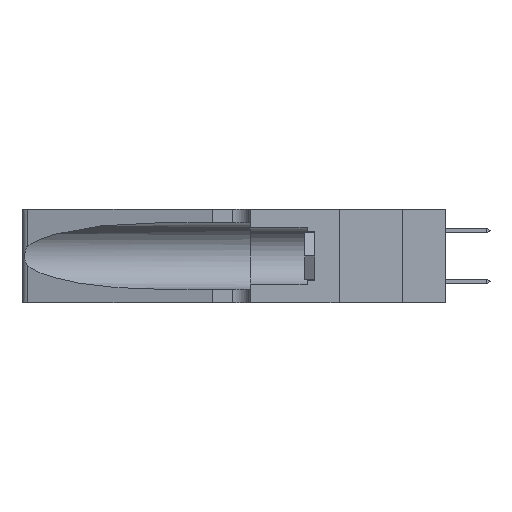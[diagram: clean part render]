
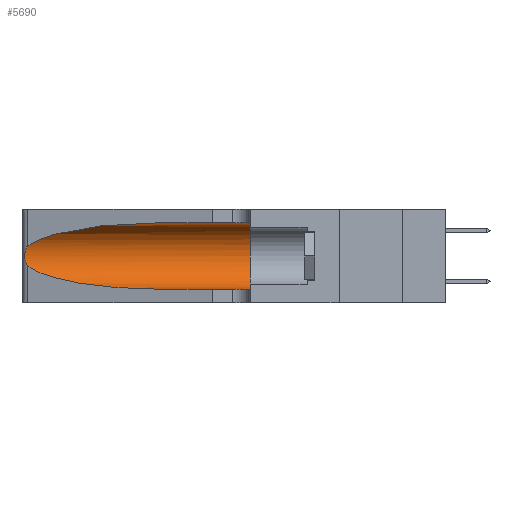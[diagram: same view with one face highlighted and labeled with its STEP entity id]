
A CAD part, left-side view. The second image highlights one B-rep face of the part: STEP entity #5690.
In plain terms, the highlighted cylindrical face has radius 3.308 mm (diameter 6.617 mm), a partial arc.
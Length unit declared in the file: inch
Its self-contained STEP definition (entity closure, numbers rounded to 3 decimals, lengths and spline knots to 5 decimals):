
#400 = VECTOR ( 'NONE', #7808, 39.37008 ) ;
#1198 = CARTESIAN_POINT ( 'NONE',  ( 0.1305, 0.72297, 0.31525 ) ) ;
#2010 = DIRECTION ( 'NONE',  ( 0., -1., 0. ) ) ;
#2629 = CYLINDRICAL_SURFACE ( 'NONE', #35287, 0.13025 ) ;
#2795 = CARTESIAN_POINT ( 'NONE',  ( 0.25555, 1.22994, 0.2215 ) ) ;
#2952 = CARTESIAN_POINT ( 'NONE',  ( 0.26017, 1.23833, 0.17102 ) ) ;
#3348 = ORIENTED_EDGE ( 'NONE', *, *, #23739, .T. ) ;
#4155 = CARTESIAN_POINT ( 'NONE',  ( 0.1305, 1.61858, 0.185 ) ) ;
#5389 = CARTESIAN_POINT ( 'NONE',  ( 0.18966, 0.96281, 0.05475 ) ) ;
#5690 = ADVANCED_FACE ( 'NONE', ( #29784 ), #2629, .F. ) ;
#6075 = DIRECTION ( 'NONE',  ( 0., 1., 0. ) ) ;
#6386 =( BOUNDED_CURVE ( )  B_SPLINE_CURVE ( 3, ( #1198, #14910, #35188, #15056 ),
 .UNSPECIFIED., .F., .T. ) 
 B_SPLINE_CURVE_WITH_KNOTS ( ( 4, 4 ),
 ( 1.5708, 2.84003 ),
 .UNSPECIFIED. ) 
 CURVE ( )  GEOMETRIC_REPRESENTATION_ITEM ( )  RATIONAL_B_SPLINE_CURVE ( ( 1., 0.87, 0.87, 1. ) ) 
 REPRESENTATION_ITEM ( '' )  );
#6492 = CARTESIAN_POINT ( 'NONE',  ( 0.25789, 1.23486, 0.15765 ) ) ;
#7808 = DIRECTION ( 'NONE',  ( 0., -1., 0. ) ) ;
#9900 = CARTESIAN_POINT ( 'NONE',  ( 0.25555, 1.22993, 0.14849 ) ) ;
#12673 = CARTESIAN_POINT ( 'NONE',  ( 0.1305, 0.35, 0.31525 ) ) ;
#12881 = VERTEX_POINT ( 'NONE', #30099 ) ;
#13112 = LINE ( 'NONE', #19233, #38848 ) ;
#14059 = ORIENTED_EDGE ( 'NONE', *, *, #23869, .T. ) ;
#14910 = CARTESIAN_POINT ( 'NONE',  ( 0.18966, 0.96281, 0.31525 ) ) ;
#15056 = CARTESIAN_POINT ( 'NONE',  ( 0.25487, 1.22718, 0.22369 ) ) ;
#16601 = CARTESIAN_POINT ( 'NONE',  ( 0.25787, 1.23484, 0.2124 ) ) ;
#16958 = AXIS2_PLACEMENT_3D ( 'NONE', #26392, #6075, #29749 ) ;
#17268 = ORIENTED_EDGE ( 'NONE', *, *, #38435, .T. ) ;
#17328 = VERTEX_POINT ( 'NONE', #18213 ) ;
#17730 = DIRECTION ( 'NONE',  ( 0., 0., -1. ) ) ;
#18213 = CARTESIAN_POINT ( 'NONE',  ( 0.25487, 1.22718, 0.14631 ) ) ;
#18695 = VERTEX_POINT ( 'NONE', #31154 ) ;
#18898 = CARTESIAN_POINT ( 'NONE',  ( 0.25487, 1.22718, 0.14631 ) ) ;
#19001 = CIRCLE ( 'NONE', #16958, 0.13025 ) ;
#19233 = CARTESIAN_POINT ( 'NONE',  ( 0.1305, 1.61858, 0.31525 ) ) ;
#19985 = CARTESIAN_POINT ( 'NONE',  ( 0.26018, 1.23835, 0.19895 ) ) ;
#20407 = VERTEX_POINT ( 'NONE', #39765 ) ;
#20425 = ORIENTED_EDGE ( 'NONE', *, *, #37039, .T. ) ;
#21340 = VERTEX_POINT ( 'NONE', #38724 ) ;
#21451 = EDGE_CURVE ( 'NONE', #12881, #41234, #13112, .T. ) ;
#23393 = CARTESIAN_POINT ( 'NONE',  ( 0.26075, 1.23896, 0.178 ) ) ;
#23739 = EDGE_CURVE ( 'NONE', #20407, #21340, #35453, .T. ) ;
#23869 = EDGE_CURVE ( 'NONE', #12881, #18695, #6386, .T. ) ;
#24214 = EDGE_LOOP ( 'NONE', ( #14059, #17268, #20425, #3348, #43461, #37735 ) ) ;
#24518 = DIRECTION ( 'NONE',  ( 0., -1., 0. ) ) ;
#26392 = CARTESIAN_POINT ( 'NONE',  ( 0.1305, 0.35, 0.185 ) ) ;
#26665 = CARTESIAN_POINT ( 'NONE',  ( 0.25487, 1.22718, 0.22369 ) ) ;
#26805 = CARTESIAN_POINT ( 'NONE',  ( 0.25856, 1.23593, 0.16098 ) ) ;
#28071 = CARTESIAN_POINT ( 'NONE',  ( 0.1305, 1.61858, 0.05475 ) ) ;
#29093 = CARTESIAN_POINT ( 'NONE',  ( 0.1305, 0.72297, 0.05475 ) ) ;
#29749 = DIRECTION ( 'NONE',  ( 0., 0., 1. ) ) ;
#29784 = FACE_OUTER_BOUND ( 'NONE', #24214, .T. ) ;
#30099 = CARTESIAN_POINT ( 'NONE',  ( 0.1305, 0.72297, 0.31525 ) ) ;
#30156 = CARTESIAN_POINT ( 'NONE',  ( 0.25639, 1.23186, 0.15144 ) ) ;
#30998 = B_SPLINE_CURVE_WITH_KNOTS ( 'NONE', 3,
 ( #26665, #2795, #36681, #16601, #40044, #19985, #43387, #23393, #2952, #26805, #6492, #30156, #9900, #33511 ),
 .UNSPECIFIED., .F., .F.,
 ( 4, 2, 2, 2, 2, 2, 4 ),
 ( 0., 0.00027, 0.00053, 0.00107, 0.0016, 0.00187, 0.00214 ),
 .UNSPECIFIED. ) ;
#31154 = CARTESIAN_POINT ( 'NONE',  ( 0.25487, 1.22718, 0.22369 ) ) ;
#31670 = EDGE_CURVE ( 'NONE', #41234, #21340, #19001, .T. ) ;
#33511 = CARTESIAN_POINT ( 'NONE',  ( 0.25487, 1.22718, 0.14631 ) ) ;
#35188 = CARTESIAN_POINT ( 'NONE',  ( 0.2373, 1.15595, 0.28018 ) ) ;
#35287 = AXIS2_PLACEMENT_3D ( 'NONE', #4155, #24518, #17730 ) ;
#35453 = LINE ( 'NONE', #28071, #400 ) ;
#35623 = CARTESIAN_POINT ( 'NONE',  ( 0.2373, 1.15595, 0.08982 ) ) ;
#36311 =( BOUNDED_CURVE ( )  B_SPLINE_CURVE ( 3, ( #18898, #35623, #5389, #29093 ),
 .UNSPECIFIED., .F., .F. ) 
 B_SPLINE_CURVE_WITH_KNOTS ( ( 4, 4 ),
 ( 3.44316, 4.71239 ),
 .UNSPECIFIED. ) 
 CURVE ( )  GEOMETRIC_REPRESENTATION_ITEM ( )  RATIONAL_B_SPLINE_CURVE ( ( 1., 0.87, 0.87, 1. ) ) 
 REPRESENTATION_ITEM ( '' )  );
#36681 = CARTESIAN_POINT ( 'NONE',  ( 0.25639, 1.23184, 0.21858 ) ) ;
#37039 = EDGE_CURVE ( 'NONE', #17328, #20407, #36311, .T. ) ;
#37735 = ORIENTED_EDGE ( 'NONE', *, *, #21451, .F. ) ;
#38435 = EDGE_CURVE ( 'NONE', #18695, #17328, #30998, .T. ) ;
#38724 = CARTESIAN_POINT ( 'NONE',  ( 0.1305, 0.35, 0.05475 ) ) ;
#38848 = VECTOR ( 'NONE', #2010, 39.37008 ) ;
#39765 = CARTESIAN_POINT ( 'NONE',  ( 0.1305, 0.72297, 0.05475 ) ) ;
#40044 = CARTESIAN_POINT ( 'NONE',  ( 0.25854, 1.2359, 0.20912 ) ) ;
#41234 = VERTEX_POINT ( 'NONE', #12673 ) ;
#43387 = CARTESIAN_POINT ( 'NONE',  ( 0.26075, 1.23896, 0.19203 ) ) ;
#43461 = ORIENTED_EDGE ( 'NONE', *, *, #31670, .F. ) ;
